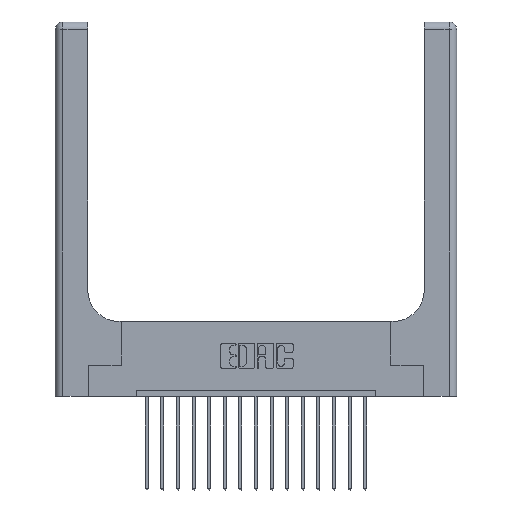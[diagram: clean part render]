
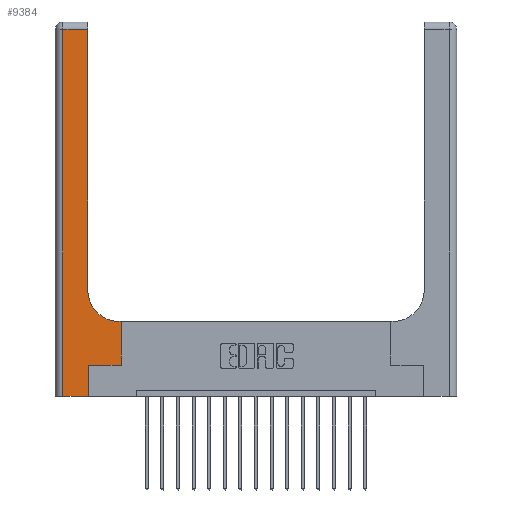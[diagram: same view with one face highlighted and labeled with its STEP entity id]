
A CAD part, top view. The second image highlights one B-rep face of the part: STEP entity #9384.
In plain terms, the highlighted planar face has unit normal (0, 0, 1).
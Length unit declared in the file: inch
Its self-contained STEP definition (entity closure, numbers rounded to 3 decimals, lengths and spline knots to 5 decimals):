
#785 = ORIENTED_EDGE ( 'NONE', *, *, #8944, .T. ) ;
#882 = CIRCLE ( 'NONE', #7154, 0.25 ) ;
#973 = CARTESIAN_POINT ( 'NONE',  ( 0.265, 0., 0.37 ) ) ;
#1289 = DIRECTION ( 'NONE',  ( 0., 0., -1. ) ) ;
#1392 = VERTEX_POINT ( 'NONE', #973 ) ;
#1592 = ORIENTED_EDGE ( 'NONE', *, *, #2058, .T. ) ;
#1716 = VECTOR ( 'NONE', #17206, 39.37008 ) ;
#1988 = LINE ( 'NONE', #16466, #9903 ) ;
#2058 = EDGE_CURVE ( 'NONE', #13389, #1392, #13895, .T. ) ;
#2526 = DIRECTION ( 'NONE',  ( -1., 0., 0. ) ) ;
#2658 = LINE ( 'NONE', #16588, #17067 ) ;
#2733 = CARTESIAN_POINT ( 'NONE',  ( 0.26, 3., 0.37 ) ) ;
#2981 = ORIENTED_EDGE ( 'NONE', *, *, #12925, .T. ) ;
#3570 = VERTEX_POINT ( 'NONE', #11160 ) ;
#3622 = CARTESIAN_POINT ( 'NONE',  ( 0.26, 0.6, 0.37 ) ) ;
#3706 = DIRECTION ( 'NONE',  ( 1., 0., 0. ) ) ;
#4104 = DIRECTION ( 'NONE',  ( -1., 0., 0. ) ) ;
#4207 = CARTESIAN_POINT ( 'NONE',  ( 0., 2.94, 0.37 ) ) ;
#4267 = ORIENTED_EDGE ( 'NONE', *, *, #9571, .T. ) ;
#4352 = CARTESIAN_POINT ( 'NONE',  ( 0.26, 0.85, 0.37 ) ) ;
#4381 = VECTOR ( 'NONE', #2526, 39.37008 ) ;
#5027 = VECTOR ( 'NONE', #12392, 39.37008 ) ;
#5160 = CARTESIAN_POINT ( 'NONE',  ( 0.51, 0.85, 0.37 ) ) ;
#5252 = VECTOR ( 'NONE', #10800, 39.37008 ) ;
#5492 = CARTESIAN_POINT ( 'NONE',  ( 0.06, 2.94, 0.37 ) ) ;
#6034 = EDGE_CURVE ( 'NONE', #8083, #13389, #1988, .T. ) ;
#6549 = DIRECTION ( 'NONE',  ( 0., 0., -1. ) ) ;
#6663 = CARTESIAN_POINT ( 'NONE',  ( 0.06, 0., 0.37 ) ) ;
#6668 = EDGE_LOOP ( 'NONE', ( #17246, #11278, #16648, #1592, #2981, #4267, #785, #10080, #7825 ) ) ;
#6712 = DIRECTION ( 'NONE',  ( -1., 0., 0. ) ) ;
#6718 = VERTEX_POINT ( 'NONE', #15170 ) ;
#7147 = CARTESIAN_POINT ( 'NONE',  ( 0.528, 0.6, 0.37 ) ) ;
#7154 = AXIS2_PLACEMENT_3D ( 'NONE', #5160, #6549, #12280 ) ;
#7766 = CARTESIAN_POINT ( 'NONE',  ( 0.265, 0.25, 0.37 ) ) ;
#7825 = ORIENTED_EDGE ( 'NONE', *, *, #14942, .T. ) ;
#8083 = VERTEX_POINT ( 'NONE', #5492 ) ;
#8156 = VERTEX_POINT ( 'NONE', #4352 ) ;
#8247 = CARTESIAN_POINT ( 'NONE',  ( 0., 0., 0.37 ) ) ;
#8591 = PLANE ( 'NONE',  #10436 ) ;
#8944 = EDGE_CURVE ( 'NONE', #6718, #11210, #18042, .T. ) ;
#9306 = DIRECTION ( 'NONE',  ( 0., -1., 0. ) ) ;
#9384 = ADVANCED_FACE ( 'NONE', ( #11250 ), #8591, .F. ) ;
#9523 = LINE ( 'NONE', #3622, #14637 ) ;
#9571 = EDGE_CURVE ( 'NONE', #11820, #6718, #2658, .T. ) ;
#9707 = CARTESIAN_POINT ( 'NONE',  ( 0.26, 2.94, 0.37 ) ) ;
#9903 = VECTOR ( 'NONE', #9306, 39.37008 ) ;
#10080 = ORIENTED_EDGE ( 'NONE', *, *, #14029, .T. ) ;
#10436 = AXIS2_PLACEMENT_3D ( 'NONE', #16989, #1289, #4104 ) ;
#10793 = LINE ( 'NONE', #16535, #11317 ) ;
#10800 = DIRECTION ( 'NONE',  ( 1., 0., 0. ) ) ;
#11073 = DIRECTION ( 'NONE',  ( 0., 1., 0. ) ) ;
#11160 = CARTESIAN_POINT ( 'NONE',  ( 0.51, 0.6, 0.37 ) ) ;
#11210 = VERTEX_POINT ( 'NONE', #7147 ) ;
#11250 = FACE_OUTER_BOUND ( 'NONE', #6668, .T. ) ;
#11278 = ORIENTED_EDGE ( 'NONE', *, *, #11922, .T. ) ;
#11317 = VECTOR ( 'NONE', #11073, 39.37008 ) ;
#11820 = VERTEX_POINT ( 'NONE', #7766 ) ;
#11922 = EDGE_CURVE ( 'NONE', #17868, #8083, #18310, .T. ) ;
#12280 = DIRECTION ( 'NONE',  ( 1., 0., 0. ) ) ;
#12392 = DIRECTION ( 'NONE',  ( 0., 1., 0. ) ) ;
#12655 = EDGE_CURVE ( 'NONE', #8156, #17868, #12685, .T. ) ;
#12685 = LINE ( 'NONE', #2733, #1716 ) ;
#12925 = EDGE_CURVE ( 'NONE', #1392, #11820, #10793, .T. ) ;
#13389 = VERTEX_POINT ( 'NONE', #6663 ) ;
#13895 = LINE ( 'NONE', #8247, #5252 ) ;
#14029 = EDGE_CURVE ( 'NONE', #11210, #3570, #9523, .T. ) ;
#14637 = VECTOR ( 'NONE', #6712, 39.37008 ) ;
#14942 = EDGE_CURVE ( 'NONE', #3570, #8156, #882, .T. ) ;
#15170 = CARTESIAN_POINT ( 'NONE',  ( 0.528, 0.25, 0.37 ) ) ;
#15214 = CARTESIAN_POINT ( 'NONE',  ( 0.528, 0.25, 0.37 ) ) ;
#16466 = CARTESIAN_POINT ( 'NONE',  ( 0.06, 3., 0.37 ) ) ;
#16535 = CARTESIAN_POINT ( 'NONE',  ( 0.265, 0., 0.37 ) ) ;
#16588 = CARTESIAN_POINT ( 'NONE',  ( 0.265, 0.25, 0.37 ) ) ;
#16648 = ORIENTED_EDGE ( 'NONE', *, *, #6034, .T. ) ;
#16989 = CARTESIAN_POINT ( 'NONE',  ( 0., 3., 0.37 ) ) ;
#17067 = VECTOR ( 'NONE', #3706, 39.37008 ) ;
#17206 = DIRECTION ( 'NONE',  ( 0., 1., 0. ) ) ;
#17246 = ORIENTED_EDGE ( 'NONE', *, *, #12655, .T. ) ;
#17868 = VERTEX_POINT ( 'NONE', #9707 ) ;
#18042 = LINE ( 'NONE', #15214, #5027 ) ;
#18310 = LINE ( 'NONE', #4207, #4381 ) ;
